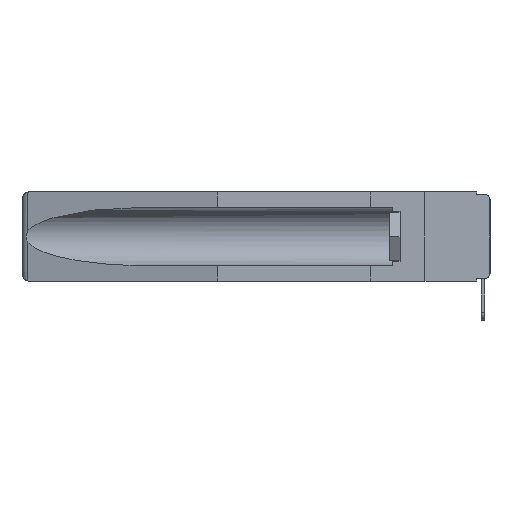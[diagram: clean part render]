
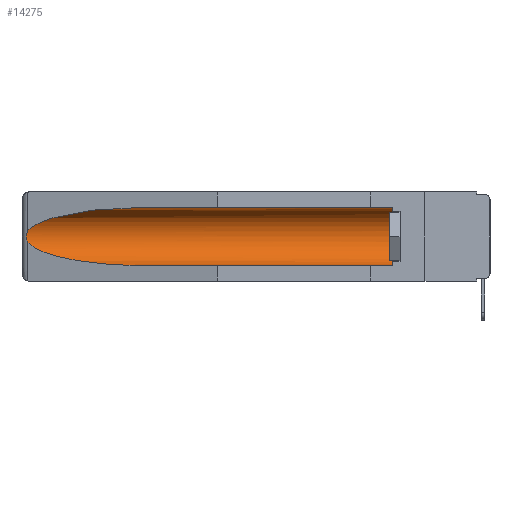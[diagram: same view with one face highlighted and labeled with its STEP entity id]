
A CAD part, left-side view. The second image highlights one B-rep face of the part: STEP entity #14275.
In plain terms, the highlighted cylindrical face has radius 2.857 mm (diameter 5.715 mm), a partial arc.
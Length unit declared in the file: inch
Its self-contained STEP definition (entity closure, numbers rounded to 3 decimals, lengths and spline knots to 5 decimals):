
#342 = EDGE_CURVE ( 'NONE', #2279, #13403, #14729, .T. ) ;
#343 = CARTESIAN_POINT ( 'NONE',  ( 0.155, 1.07973, -0.284 ) ) ;
#1246 = EDGE_LOOP ( 'NONE', ( #15216, #9874, #6345, #11908, #17020, #16964 ) ) ;
#1595 = CARTESIAN_POINT ( 'NONE',  ( 0.2675, 1.53308, -0.16763 ) ) ;
#1616 = LINE ( 'NONE', #3558, #17405 ) ;
#2226 = B_SPLINE_CURVE_WITH_KNOTS ( 'NONE', 3,
 ( #3066, #6946, #7186, #8342, #1595, #15059, #10983, #4356, #11227, #4412 ),
 .UNSPECIFIED., .F., .F.,
 ( 4, 2, 2, 2, 4 ),
 ( 0., 0.00029, 0.00058, 0.00087, 0.00117 ),
 .UNSPECIFIED. ) ;
#2256 = DIRECTION ( 'NONE',  ( 0., 1., 0. ) ) ;
#2279 = VERTEX_POINT ( 'NONE', #5601 ) ;
#2488 = VERTEX_POINT ( 'NONE', #15692 ) ;
#2517 = DIRECTION ( 'NONE',  ( 0., 1., 0. ) ) ;
#2812 = LINE ( 'NONE', #7560, #4299 ) ;
#3066 = CARTESIAN_POINT ( 'NONE',  ( 0.26537, 1.52718, -0.14972 ) ) ;
#3558 = CARTESIAN_POINT ( 'NONE',  ( 0.155, -0.30754, -0.284 ) ) ;
#4299 = VECTOR ( 'NONE', #4621, 39.37008 ) ;
#4356 = CARTESIAN_POINT ( 'NONE',  ( 0.26655, 1.53094, -0.18657 ) ) ;
#4412 = CARTESIAN_POINT ( 'NONE',  ( 0.26537, 1.52718, -0.19328 ) ) ;
#4582 =( BOUNDED_CURVE ( )  B_SPLINE_CURVE ( 3, ( #12628, #13980, #16704, #16763 ),
 .UNSPECIFIED., .F., .F. ) 
 B_SPLINE_CURVE_WITH_KNOTS ( ( 4, 4 ),
 ( 4.71239, 6.08839 ),
 .UNSPECIFIED. ) 
 CURVE ( )  GEOMETRIC_REPRESENTATION_ITEM ( )  RATIONAL_B_SPLINE_CURVE ( ( 1., 0.848, 0.848, 1. ) ) 
 REPRESENTATION_ITEM ( '' )  );
#4621 = DIRECTION ( 'NONE',  ( 0., 1., 0. ) ) ;
#5171 = AXIS2_PLACEMENT_3D ( 'NONE', #17228, #2517, #11985 ) ;
#5601 = CARTESIAN_POINT ( 'NONE',  ( 0.26537, 1.52718, -0.19328 ) ) ;
#5622 = VERTEX_POINT ( 'NONE', #14241 ) ;
#6345 = ORIENTED_EDGE ( 'NONE', *, *, #342, .T. ) ;
#6549 = EDGE_CURVE ( 'NONE', #8141, #13403, #1616, .T. ) ;
#6946 = CARTESIAN_POINT ( 'NONE',  ( 0.26597, 1.52961, -0.15275 ) ) ;
#7186 = CARTESIAN_POINT ( 'NONE',  ( 0.26654, 1.53092, -0.15636 ) ) ;
#7560 = CARTESIAN_POINT ( 'NONE',  ( 0.155, -0.30754, -0.059 ) ) ;
#8141 = VERTEX_POINT ( 'NONE', #8812 ) ;
#8342 = CARTESIAN_POINT ( 'NONE',  ( 0.2673, 1.5327, -0.16383 ) ) ;
#8619 = EDGE_CURVE ( 'NONE', #5622, #2488, #4582, .T. ) ;
#8812 = CARTESIAN_POINT ( 'NONE',  ( 0.155, 0.126, -0.284 ) ) ;
#9676 = CYLINDRICAL_SURFACE ( 'NONE', #5171, 0.1125 ) ;
#9874 = ORIENTED_EDGE ( 'NONE', *, *, #12133, .T. ) ;
#10105 = FACE_OUTER_BOUND ( 'NONE', #1246, .T. ) ;
#10114 = CARTESIAN_POINT ( 'NONE',  ( 0.26537, 1.52718, -0.19328 ) ) ;
#10304 = EDGE_CURVE ( 'NONE', #8141, #11300, #10523, .T. ) ;
#10523 = CIRCLE ( 'NONE', #15271, 0.1125 ) ;
#10983 = CARTESIAN_POINT ( 'NONE',  ( 0.2673, 1.53269, -0.17917 ) ) ;
#11046 = CARTESIAN_POINT ( 'NONE',  ( 0.155, 0.126, -0.059 ) ) ;
#11227 = CARTESIAN_POINT ( 'NONE',  ( 0.26597, 1.5296, -0.19026 ) ) ;
#11300 = VERTEX_POINT ( 'NONE', #11046 ) ;
#11908 = ORIENTED_EDGE ( 'NONE', *, *, #6549, .F. ) ;
#11985 = DIRECTION ( 'NONE',  ( 0., 0., 1. ) ) ;
#12133 = EDGE_CURVE ( 'NONE', #2488, #2279, #2226, .T. ) ;
#12628 = CARTESIAN_POINT ( 'NONE',  ( 0.155, 1.07973, -0.059 ) ) ;
#12845 = CARTESIAN_POINT ( 'NONE',  ( 0.155, 1.07973, -0.284 ) ) ;
#12892 = EDGE_CURVE ( 'NONE', #11300, #5622, #2812, .T. ) ;
#13403 = VERTEX_POINT ( 'NONE', #343 ) ;
#13980 = CARTESIAN_POINT ( 'NONE',  ( 0.21114, 1.30732, -0.059 ) ) ;
#14241 = CARTESIAN_POINT ( 'NONE',  ( 0.155, 1.07973, -0.059 ) ) ;
#14275 = ADVANCED_FACE ( 'NONE', ( #10105 ), #9676, .F. ) ;
#14337 = CARTESIAN_POINT ( 'NONE',  ( 0.155, 0.126, -0.1715 ) ) ;
#14729 =( BOUNDED_CURVE ( )  B_SPLINE_CURVE ( 3, ( #10114, #16959, #16851, #12845 ),
 .UNSPECIFIED., .F., .T. ) 
 B_SPLINE_CURVE_WITH_KNOTS ( ( 4, 4 ),
 ( 0.1948, 1.5708 ),
 .UNSPECIFIED. ) 
 CURVE ( )  GEOMETRIC_REPRESENTATION_ITEM ( )  RATIONAL_B_SPLINE_CURVE ( ( 1., 0.848, 0.848, 1. ) ) 
 REPRESENTATION_ITEM ( '' )  );
#15059 = CARTESIAN_POINT ( 'NONE',  ( 0.2675, 1.53308, -0.17534 ) ) ;
#15216 = ORIENTED_EDGE ( 'NONE', *, *, #8619, .T. ) ;
#15271 = AXIS2_PLACEMENT_3D ( 'NONE', #14337, #15624, #16988 ) ;
#15624 = DIRECTION ( 'NONE',  ( 0., -1., 0. ) ) ;
#15692 = CARTESIAN_POINT ( 'NONE',  ( 0.26537, 1.52718, -0.14972 ) ) ;
#16704 = CARTESIAN_POINT ( 'NONE',  ( 0.25451, 1.48313, -0.09465 ) ) ;
#16763 = CARTESIAN_POINT ( 'NONE',  ( 0.26537, 1.52718, -0.14972 ) ) ;
#16851 = CARTESIAN_POINT ( 'NONE',  ( 0.21114, 1.30732, -0.284 ) ) ;
#16959 = CARTESIAN_POINT ( 'NONE',  ( 0.25451, 1.48313, -0.24835 ) ) ;
#16964 = ORIENTED_EDGE ( 'NONE', *, *, #12892, .T. ) ;
#16988 = DIRECTION ( 'NONE',  ( 0., 0., 1. ) ) ;
#17020 = ORIENTED_EDGE ( 'NONE', *, *, #10304, .T. ) ;
#17228 = CARTESIAN_POINT ( 'NONE',  ( 0.155, -0.30754, -0.1715 ) ) ;
#17405 = VECTOR ( 'NONE', #2256, 39.37008 ) ;
